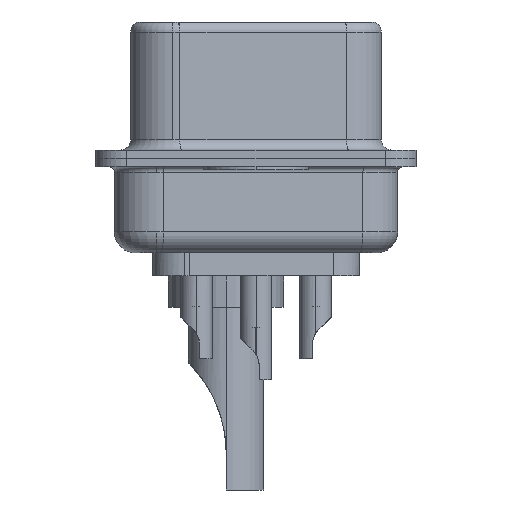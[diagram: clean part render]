
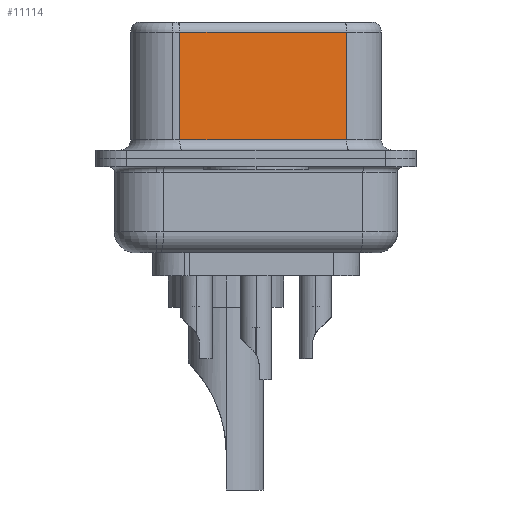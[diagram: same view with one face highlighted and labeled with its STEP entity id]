
A CAD part, left-side view. The second image highlights one B-rep face of the part: STEP entity #11114.
In plain terms, the highlighted planar face has unit normal (-0.985, -0.174, 0).
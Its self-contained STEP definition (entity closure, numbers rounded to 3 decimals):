
#1222 = EDGE_CURVE ( 'NONE', #16834, #18085, #25421, .T. ) ;
#1784 = CARTESIAN_POINT ( 'NONE',  ( 5.132, -4.322, 6.02 ) ) ;
#3722 = CARTESIAN_POINT ( 'NONE',  ( 5.132, -4.322, 0.9 ) ) ;
#3808 = DIRECTION ( 'NONE',  ( 0.985, 0.174, 0. ) ) ;
#9563 = EDGE_CURVE ( 'NONE', #20360, #16834, #17209, .T. ) ;
#10432 = VECTOR ( 'NONE', #16546, 1000. ) ;
#10482 = CARTESIAN_POINT ( 'NONE',  ( 5.132, -4.322, 6.02 ) ) ;
#11114 = ADVANCED_FACE ( 'NONE', ( #19471 ), #12378, .F. ) ;
#11380 = VECTOR ( 'NONE', #23275, 1000. ) ;
#11718 = CARTESIAN_POINT ( 'NONE',  ( 3.73, 3.628, 6.02 ) ) ;
#12378 = PLANE ( 'NONE',  #24666 ) ;
#12791 = LINE ( 'NONE', #3722, #10432 ) ;
#14699 = CARTESIAN_POINT ( 'NONE',  ( 5.132, -4.322, 6.52 ) ) ;
#15072 = ORIENTED_EDGE ( 'NONE', *, *, #1222, .T. ) ;
#16229 = EDGE_LOOP ( 'NONE', ( #17460, #16245, #15072, #18878 ) ) ;
#16245 = ORIENTED_EDGE ( 'NONE', *, *, #9563, .T. ) ;
#16546 = DIRECTION ( 'NONE',  ( 0.174, -0.985, 0. ) ) ;
#16622 = CARTESIAN_POINT ( 'NONE',  ( 3.73, 3.628, 0.9 ) ) ;
#16673 = VECTOR ( 'NONE', #23877, 1000. ) ;
#16834 = VERTEX_POINT ( 'NONE', #11718 ) ;
#17209 = LINE ( 'NONE', #1784, #11380 ) ;
#17460 = ORIENTED_EDGE ( 'NONE', *, *, #22548, .F. ) ;
#18085 = VERTEX_POINT ( 'NONE', #16622 ) ;
#18878 = ORIENTED_EDGE ( 'NONE', *, *, #21687, .T. ) ;
#19471 = FACE_OUTER_BOUND ( 'NONE', #16229, .T. ) ;
#20360 = VERTEX_POINT ( 'NONE', #10482 ) ;
#21687 = EDGE_CURVE ( 'NONE', #18085, #22444, #12791, .T. ) ;
#21858 = CARTESIAN_POINT ( 'NONE',  ( 5.132, -4.322, 6.52 ) ) ;
#21962 = LINE ( 'NONE', #21858, #24332 ) ;
#22444 = VERTEX_POINT ( 'NONE', #25349 ) ;
#22548 = EDGE_CURVE ( 'NONE', #20360, #22444, #21962, .T. ) ;
#23275 = DIRECTION ( 'NONE',  ( -0.174, 0.985, 0. ) ) ;
#23404 = DIRECTION ( 'NONE',  ( -0.174, 0.985, 0. ) ) ;
#23499 = CARTESIAN_POINT ( 'NONE',  ( 3.73, 3.628, 6.52 ) ) ;
#23877 = DIRECTION ( 'NONE',  ( 0., 0., -1. ) ) ;
#24332 = VECTOR ( 'NONE', #26106, 1000. ) ;
#24666 = AXIS2_PLACEMENT_3D ( 'NONE', #14699, #3808, #23404 ) ;
#25349 = CARTESIAN_POINT ( 'NONE',  ( 5.132, -4.322, 0.9 ) ) ;
#25421 = LINE ( 'NONE', #23499, #16673 ) ;
#26106 = DIRECTION ( 'NONE',  ( 0., 0., -1. ) ) ;
